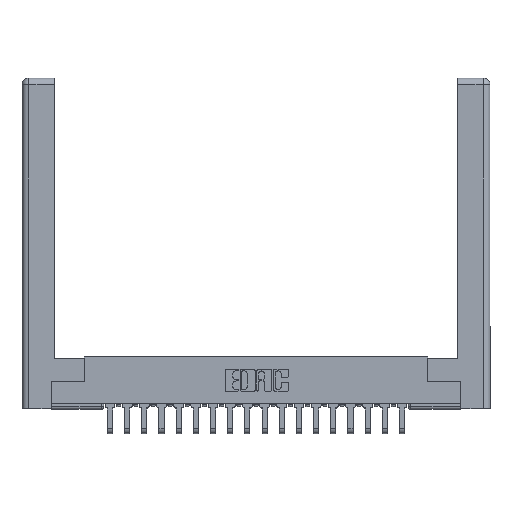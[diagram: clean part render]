
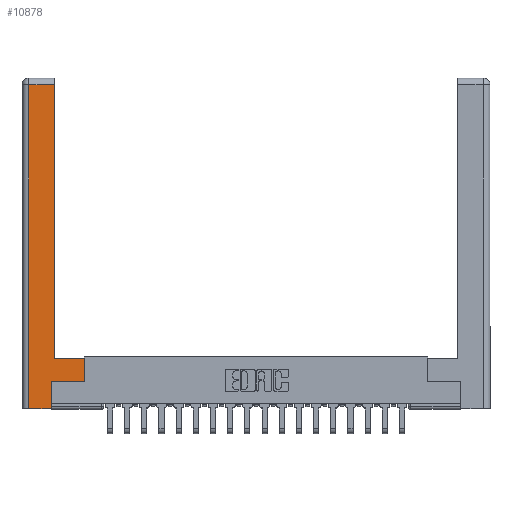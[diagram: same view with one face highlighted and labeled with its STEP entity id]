
A CAD part, top view. The second image highlights one B-rep face of the part: STEP entity #10878.
In plain terms, the highlighted planar face has unit normal (0, 0, 1).
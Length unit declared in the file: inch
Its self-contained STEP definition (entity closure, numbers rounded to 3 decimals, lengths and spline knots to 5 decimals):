
#202 = DIRECTION ( 'NONE',  ( 1., 0., 0. ) ) ;
#353 = EDGE_CURVE ( 'NONE', #4349, #12232, #9443, .T. ) ;
#369 = VERTEX_POINT ( 'NONE', #12599 ) ;
#372 = FACE_OUTER_BOUND ( 'NONE', #19605, .T. ) ;
#1146 = VERTEX_POINT ( 'NONE', #13715 ) ;
#1205 = ORIENTED_EDGE ( 'NONE', *, *, #9108, .T. ) ;
#1759 = CARTESIAN_POINT ( 'NONE',  ( 0.0615, 0., 0. ) ) ;
#1899 = CARTESIAN_POINT ( 'NONE',  ( 0.265, 0., 0. ) ) ;
#1936 = LINE ( 'NONE', #17827, #8969 ) ;
#2084 = DIRECTION ( 'NONE',  ( 1., 0., 0. ) ) ;
#2111 = EDGE_CURVE ( 'NONE', #369, #22623, #14317, .T. ) ;
#2219 = ORIENTED_EDGE ( 'NONE', *, *, #9540, .T. ) ;
#3759 = CARTESIAN_POINT ( 'NONE',  ( 0.295, 0.45, 0. ) ) ;
#3858 = ORIENTED_EDGE ( 'NONE', *, *, #353, .T. ) ;
#4349 = VERTEX_POINT ( 'NONE', #1759 ) ;
#5000 = LINE ( 'NONE', #21270, #14860 ) ;
#5454 = VECTOR ( 'NONE', #15722, 39.37008 ) ;
#5948 = CARTESIAN_POINT ( 'NONE',  ( 0.0615, 0., 0. ) ) ;
#6117 = VECTOR ( 'NONE', #18019, 39.37008 ) ;
#6428 = EDGE_CURVE ( 'NONE', #12232, #369, #22735, .T. ) ;
#7340 = CARTESIAN_POINT ( 'NONE',  ( 0.295, 3., 0. ) ) ;
#8151 = CARTESIAN_POINT ( 'NONE',  ( 0.565, 0.45, 0. ) ) ;
#8969 = VECTOR ( 'NONE', #19822, 39.37008 ) ;
#9108 = EDGE_CURVE ( 'NONE', #9906, #12320, #12995, .T. ) ;
#9136 = ORIENTED_EDGE ( 'NONE', *, *, #2111, .T. ) ;
#9183 = CARTESIAN_POINT ( 'NONE',  ( 0.565, 0.245, 0. ) ) ;
#9443 = LINE ( 'NONE', #20089, #21789 ) ;
#9540 = EDGE_CURVE ( 'NONE', #12320, #1146, #21371, .T. ) ;
#9906 = VERTEX_POINT ( 'NONE', #8151 ) ;
#9978 = ORIENTED_EDGE ( 'NONE', *, *, #14179, .T. ) ;
#10878 = ADVANCED_FACE ( 'NONE', ( #372 ), #12733, .F. ) ;
#12232 = VERTEX_POINT ( 'NONE', #1899 ) ;
#12320 = VERTEX_POINT ( 'NONE', #12763 ) ;
#12599 = CARTESIAN_POINT ( 'NONE',  ( 0.265, 0.245, 0. ) ) ;
#12727 = DIRECTION ( 'NONE',  ( 0., 1., 0. ) ) ;
#12733 = PLANE ( 'NONE',  #15509 ) ;
#12735 = LINE ( 'NONE', #5948, #22588 ) ;
#12763 = CARTESIAN_POINT ( 'NONE',  ( 0.295, 0.45, 0. ) ) ;
#12843 = DIRECTION ( 'NONE',  ( -1., 0., 0. ) ) ;
#12995 = LINE ( 'NONE', #3759, #6117 ) ;
#13114 = CARTESIAN_POINT ( 'NONE',  ( 0.0615, 2.94, 0. ) ) ;
#13715 = CARTESIAN_POINT ( 'NONE',  ( 0.295, 2.94, 0. ) ) ;
#14179 = EDGE_CURVE ( 'NONE', #1146, #18679, #5000, .T. ) ;
#14240 = DIRECTION ( 'NONE',  ( 0., 0., -1. ) ) ;
#14317 = LINE ( 'NONE', #9183, #18240 ) ;
#14715 = EDGE_CURVE ( 'NONE', #22623, #9906, #1936, .T. ) ;
#14860 = VECTOR ( 'NONE', #19402, 39.37008 ) ;
#15248 = ORIENTED_EDGE ( 'NONE', *, *, #14715, .T. ) ;
#15509 = AXIS2_PLACEMENT_3D ( 'NONE', #19867, #14240, #12843 ) ;
#15722 = DIRECTION ( 'NONE',  ( 0., 1., 0. ) ) ;
#16705 = DIRECTION ( 'NONE',  ( 0., -1., 0. ) ) ;
#17827 = CARTESIAN_POINT ( 'NONE',  ( 0.565, 0.45, 0. ) ) ;
#18019 = DIRECTION ( 'NONE',  ( -1., 0., 0. ) ) ;
#18240 = VECTOR ( 'NONE', #202, 39.37008 ) ;
#18679 = VERTEX_POINT ( 'NONE', #13114 ) ;
#19263 = ORIENTED_EDGE ( 'NONE', *, *, #21801, .T. ) ;
#19402 = DIRECTION ( 'NONE',  ( -1., 0., 0. ) ) ;
#19605 = EDGE_LOOP ( 'NONE', ( #2219, #9978, #19263, #3858, #21115, #9136, #15248, #1205 ) ) ;
#19822 = DIRECTION ( 'NONE',  ( 0., 1., 0. ) ) ;
#19867 = CARTESIAN_POINT ( 'NONE',  ( 0., 0., 0. ) ) ;
#20089 = CARTESIAN_POINT ( 'NONE',  ( 0.265, 0., 0. ) ) ;
#21073 = VECTOR ( 'NONE', #12727, 39.37008 ) ;
#21115 = ORIENTED_EDGE ( 'NONE', *, *, #6428, .T. ) ;
#21270 = CARTESIAN_POINT ( 'NONE',  ( 0.0615, 2.94, 0. ) ) ;
#21371 = LINE ( 'NONE', #7340, #21073 ) ;
#21789 = VECTOR ( 'NONE', #2084, 39.37008 ) ;
#21801 = EDGE_CURVE ( 'NONE', #18679, #4349, #12735, .T. ) ;
#22000 = CARTESIAN_POINT ( 'NONE',  ( 0.565, 0.245, 0. ) ) ;
#22588 = VECTOR ( 'NONE', #16705, 39.37008 ) ;
#22623 = VERTEX_POINT ( 'NONE', #22000 ) ;
#22735 = LINE ( 'NONE', #22957, #5454 ) ;
#22957 = CARTESIAN_POINT ( 'NONE',  ( 0.265, 0.245, 0. ) ) ;
